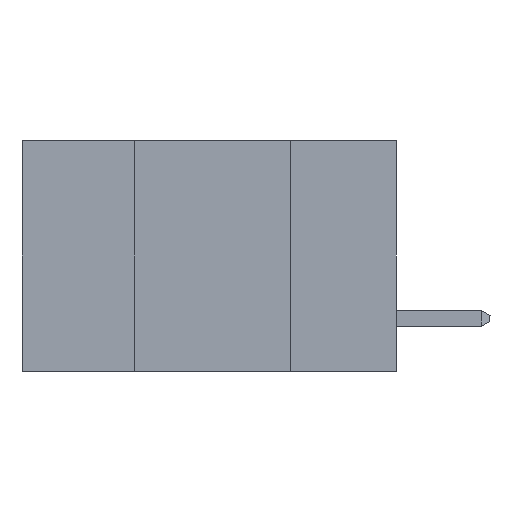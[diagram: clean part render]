
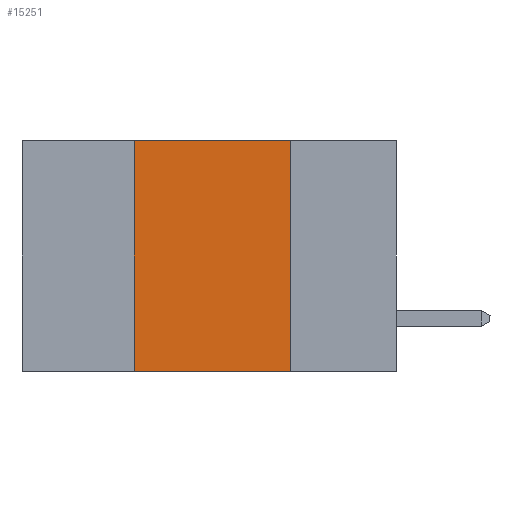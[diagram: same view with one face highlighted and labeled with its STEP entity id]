
A CAD part, left-side view. The second image highlights one B-rep face of the part: STEP entity #15251.
In plain terms, the highlighted planar face has unit normal (-1, 0, 0).
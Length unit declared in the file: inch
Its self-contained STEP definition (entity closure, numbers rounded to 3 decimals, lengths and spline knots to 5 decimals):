
#191 = VECTOR ( 'NONE', #18534, 39.37008 ) ;
#625 = LINE ( 'NONE', #6885, #6616 ) ;
#780 = VERTEX_POINT ( 'NONE', #22385 ) ;
#1265 = VERTEX_POINT ( 'NONE', #16882 ) ;
#2326 = ORIENTED_EDGE ( 'NONE', *, *, #12202, .F. ) ;
#2706 = DIRECTION ( 'NONE',  ( 1., 0., 0. ) ) ;
#4614 = CARTESIAN_POINT ( 'NONE',  ( 0., 0.42, -0.37 ) ) ;
#5843 = ORIENTED_EDGE ( 'NONE', *, *, #24398, .F. ) ;
#6139 = ORIENTED_EDGE ( 'NONE', *, *, #17450, .F. ) ;
#6616 = VECTOR ( 'NONE', #22646, 39.37008 ) ;
#6761 = CARTESIAN_POINT ( 'NONE',  ( 0., 0.42, 0. ) ) ;
#6885 = CARTESIAN_POINT ( 'NONE',  ( 0., 0.6, 0. ) ) ;
#8484 = CARTESIAN_POINT ( 'NONE',  ( 0., 0.17, -0.37 ) ) ;
#9284 = VECTOR ( 'NONE', #20305, 39.37008 ) ;
#9485 = DIRECTION ( 'NONE',  ( 0., -1., 0. ) ) ;
#9932 = LINE ( 'NONE', #8484, #9284 ) ;
#12202 = EDGE_CURVE ( 'NONE', #19767, #1265, #625, .T. ) ;
#13822 = LINE ( 'NONE', #23196, #14460 ) ;
#13863 = EDGE_LOOP ( 'NONE', ( #5843, #2326, #6139, #21899 ) ) ;
#14460 = VECTOR ( 'NONE', #9485, 39.37008 ) ;
#14742 = PLANE ( 'NONE',  #25382 ) ;
#15251 = ADVANCED_FACE ( 'NONE', ( #16155 ), #14742, .F. ) ;
#16155 = FACE_OUTER_BOUND ( 'NONE', #13863, .T. ) ;
#16176 = LINE ( 'NONE', #4614, #191 ) ;
#16710 = DIRECTION ( 'NONE',  ( 0., 0., -1. ) ) ;
#16882 = CARTESIAN_POINT ( 'NONE',  ( 0., 0.17, 0. ) ) ;
#17450 = EDGE_CURVE ( 'NONE', #21565, #19767, #16176, .T. ) ;
#18037 = CARTESIAN_POINT ( 'NONE',  ( 0., 0.42, -0.37 ) ) ;
#18534 = DIRECTION ( 'NONE',  ( 0., 0., 1. ) ) ;
#19767 = VERTEX_POINT ( 'NONE', #6761 ) ;
#20305 = DIRECTION ( 'NONE',  ( 0., 0., -1. ) ) ;
#21357 = EDGE_CURVE ( 'NONE', #21565, #780, #13822, .T. ) ;
#21565 = VERTEX_POINT ( 'NONE', #18037 ) ;
#21899 = ORIENTED_EDGE ( 'NONE', *, *, #21357, .T. ) ;
#22385 = CARTESIAN_POINT ( 'NONE',  ( 0., 0.17, -0.37 ) ) ;
#22466 = CARTESIAN_POINT ( 'NONE',  ( 0., 0.6, 0. ) ) ;
#22646 = DIRECTION ( 'NONE',  ( 0., -1., 0. ) ) ;
#23196 = CARTESIAN_POINT ( 'NONE',  ( 0., 0.6, -0.37 ) ) ;
#24398 = EDGE_CURVE ( 'NONE', #1265, #780, #9932, .T. ) ;
#25382 = AXIS2_PLACEMENT_3D ( 'NONE', #22466, #2706, #16710 ) ;
